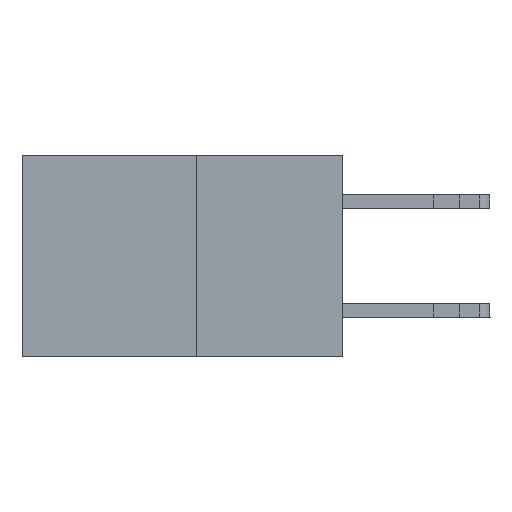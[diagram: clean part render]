
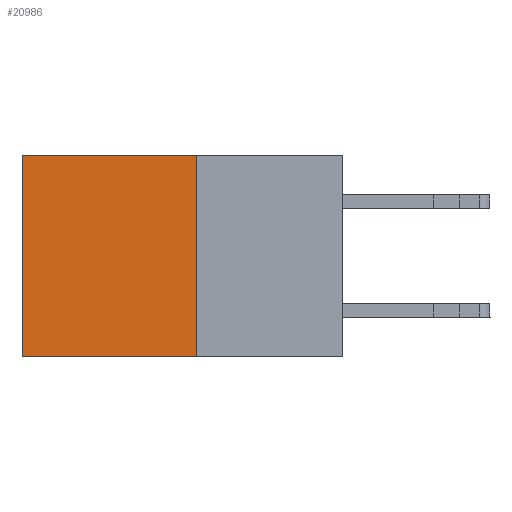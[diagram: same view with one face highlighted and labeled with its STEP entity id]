
A CAD part, left-side view. The second image highlights one B-rep face of the part: STEP entity #20986.
In plain terms, the highlighted planar face has unit normal (-1, 0, 0).
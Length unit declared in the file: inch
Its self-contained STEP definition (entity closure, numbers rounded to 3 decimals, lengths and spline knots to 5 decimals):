
#2163 = VECTOR ( 'NONE', #9360, 39.37008 ) ;
#2546 = EDGE_CURVE ( 'NONE', #11780, #9585, #4279, .T. ) ;
#4084 = CARTESIAN_POINT ( 'NONE',  ( 0.277, 0.27, -0.37 ) ) ;
#4279 = LINE ( 'NONE', #18480, #23472 ) ;
#5962 = EDGE_LOOP ( 'NONE', ( #7151, #16781, #22402, #10055 ) ) ;
#6059 = VERTEX_POINT ( 'NONE', #20638 ) ;
#6092 = VERTEX_POINT ( 'NONE', #20726 ) ;
#6136 = DIRECTION ( 'NONE',  ( 0., 0., -1. ) ) ;
#7151 = ORIENTED_EDGE ( 'NONE', *, *, #10528, .T. ) ;
#8127 = LINE ( 'NONE', #22987, #2163 ) ;
#8586 = EDGE_CURVE ( 'NONE', #11780, #6092, #22282, .T. ) ;
#9360 = DIRECTION ( 'NONE',  ( 0., 1., 0. ) ) ;
#9585 = VERTEX_POINT ( 'NONE', #21893 ) ;
#10055 = ORIENTED_EDGE ( 'NONE', *, *, #2546, .T. ) ;
#10412 = CARTESIAN_POINT ( 'NONE',  ( 0.277, 0.27, -0.37 ) ) ;
#10528 = EDGE_CURVE ( 'NONE', #9585, #6059, #24620, .T. ) ;
#11316 = EDGE_CURVE ( 'NONE', #6092, #6059, #8127, .T. ) ;
#11780 = VERTEX_POINT ( 'NONE', #13033 ) ;
#12381 = DIRECTION ( 'NONE',  ( 0., 0., -1. ) ) ;
#12549 = VECTOR ( 'NONE', #6136, 39.37008 ) ;
#13033 = CARTESIAN_POINT ( 'NONE',  ( 0.277, 0.27, 0. ) ) ;
#13088 = CARTESIAN_POINT ( 'NONE',  ( 0.277, 0.59, -0.37 ) ) ;
#15363 = DIRECTION ( 'NONE',  ( 0., 1., 0. ) ) ;
#16781 = ORIENTED_EDGE ( 'NONE', *, *, #11316, .F. ) ;
#18480 = CARTESIAN_POINT ( 'NONE',  ( 0.277, 0.27, 0. ) ) ;
#19552 = VECTOR ( 'NONE', #24693, 39.37008 ) ;
#20146 = PLANE ( 'NONE',  #23791 ) ;
#20638 = CARTESIAN_POINT ( 'NONE',  ( 0.277, 0.59, -0.37 ) ) ;
#20726 = CARTESIAN_POINT ( 'NONE',  ( 0.277, 0.27, -0.37 ) ) ;
#20986 = ADVANCED_FACE ( 'NONE', ( #22341 ), #20146, .F. ) ;
#21893 = CARTESIAN_POINT ( 'NONE',  ( 0.277, 0.59, 0. ) ) ;
#22282 = LINE ( 'NONE', #4084, #12549 ) ;
#22341 = FACE_OUTER_BOUND ( 'NONE', #5962, .T. ) ;
#22402 = ORIENTED_EDGE ( 'NONE', *, *, #8586, .F. ) ;
#22987 = CARTESIAN_POINT ( 'NONE',  ( 0.277, 0.27, -0.37 ) ) ;
#23472 = VECTOR ( 'NONE', #15363, 39.37008 ) ;
#23791 = AXIS2_PLACEMENT_3D ( 'NONE', #10412, #24008, #12381 ) ;
#24008 = DIRECTION ( 'NONE',  ( 1., 0., 0. ) ) ;
#24620 = LINE ( 'NONE', #13088, #19552 ) ;
#24693 = DIRECTION ( 'NONE',  ( 0., 0., -1. ) ) ;
